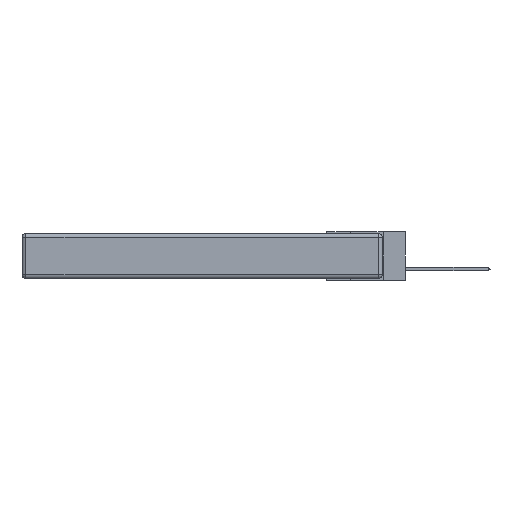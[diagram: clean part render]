
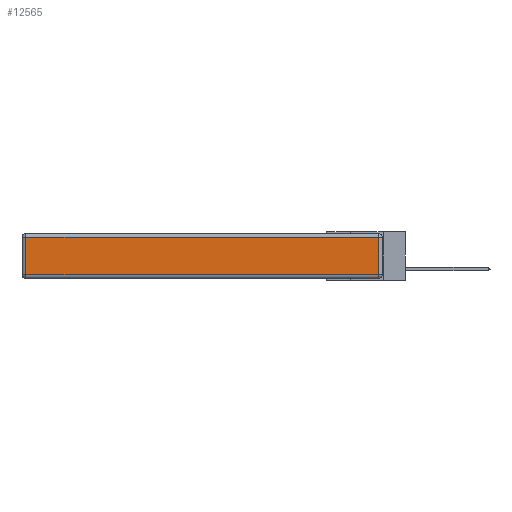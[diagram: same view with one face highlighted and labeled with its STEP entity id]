
A CAD part, left-side view. The second image highlights one B-rep face of the part: STEP entity #12565.
In plain terms, the highlighted planar face has unit normal (-1, 0, 0).
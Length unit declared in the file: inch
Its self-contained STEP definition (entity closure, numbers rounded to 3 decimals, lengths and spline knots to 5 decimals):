
#643 = CARTESIAN_POINT ( 'NONE',  ( 0., 0., -0.313 ) ) ;
#1876 = ORIENTED_EDGE ( 'NONE', *, *, #9236, .T. ) ;
#2008 = ORIENTED_EDGE ( 'NONE', *, *, #4017, .T. ) ;
#2500 = EDGE_LOOP ( 'NONE', ( #2008, #20349, #1876, #14589 ) ) ;
#2587 = FACE_OUTER_BOUND ( 'NONE', #2500, .T. ) ;
#3212 = DIRECTION ( 'NONE',  ( -1., 0., 0. ) ) ;
#4017 = EDGE_CURVE ( 'NONE', #10712, #19300, #12367, .T. ) ;
#5515 = CARTESIAN_POINT ( 'NONE',  ( 0., 0.03, -0.03 ) ) ;
#7193 = DIRECTION ( 'NONE',  ( 0., 0., 1. ) ) ;
#7510 = VECTOR ( 'NONE', #19591, 39.37008 ) ;
#7679 = VECTOR ( 'NONE', #12876, 39.37008 ) ;
#8700 = CARTESIAN_POINT ( 'NONE',  ( 0., 0.03, -0.343 ) ) ;
#9236 = EDGE_CURVE ( 'NONE', #10469, #9492, #11831, .T. ) ;
#9492 = VERTEX_POINT ( 'NONE', #13045 ) ;
#10469 = VERTEX_POINT ( 'NONE', #5515 ) ;
#10712 = VERTEX_POINT ( 'NONE', #23506 ) ;
#11751 = EDGE_CURVE ( 'NONE', #19300, #10469, #18792, .T. ) ;
#11831 = LINE ( 'NONE', #15750, #7510 ) ;
#12367 = LINE ( 'NONE', #643, #15159 ) ;
#12565 = ADVANCED_FACE ( 'NONE', ( #2587 ), #17038, .T. ) ;
#12876 = DIRECTION ( 'NONE',  ( 0., 0., 1. ) ) ;
#13045 = CARTESIAN_POINT ( 'NONE',  ( 0., 2.72, -0.03 ) ) ;
#13525 = DIRECTION ( 'NONE',  ( 0., 0., -1. ) ) ;
#14589 = ORIENTED_EDGE ( 'NONE', *, *, #22337, .T. ) ;
#15159 = VECTOR ( 'NONE', #18166, 39.37008 ) ;
#15750 = CARTESIAN_POINT ( 'NONE',  ( 0., 2.75, -0.03 ) ) ;
#17038 = PLANE ( 'NONE',  #22992 ) ;
#18001 = CARTESIAN_POINT ( 'NONE',  ( 0., 2.72, -0.343 ) ) ;
#18166 = DIRECTION ( 'NONE',  ( 0., -1., 0. ) ) ;
#18349 = VECTOR ( 'NONE', #13525, 39.37008 ) ;
#18792 = LINE ( 'NONE', #8700, #7679 ) ;
#19300 = VERTEX_POINT ( 'NONE', #21171 ) ;
#19591 = DIRECTION ( 'NONE',  ( 0., 1., 0. ) ) ;
#20349 = ORIENTED_EDGE ( 'NONE', *, *, #11751, .T. ) ;
#21171 = CARTESIAN_POINT ( 'NONE',  ( 0., 0.03, -0.313 ) ) ;
#22337 = EDGE_CURVE ( 'NONE', #9492, #10712, #22982, .T. ) ;
#22710 = CARTESIAN_POINT ( 'NONE',  ( 0., 0., -0.343 ) ) ;
#22982 = LINE ( 'NONE', #18001, #18349 ) ;
#22992 = AXIS2_PLACEMENT_3D ( 'NONE', #22710, #3212, #7193 ) ;
#23506 = CARTESIAN_POINT ( 'NONE',  ( 0., 2.72, -0.313 ) ) ;
